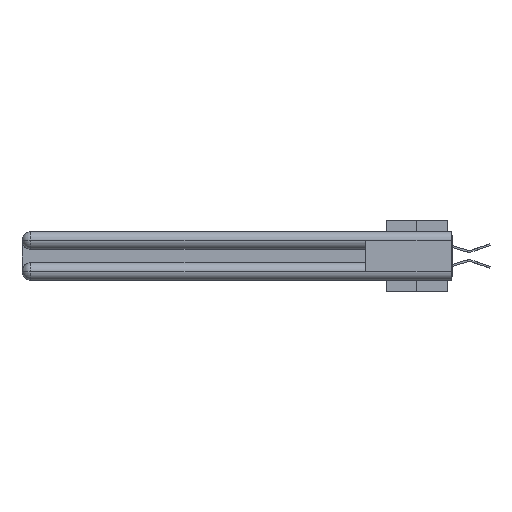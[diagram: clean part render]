
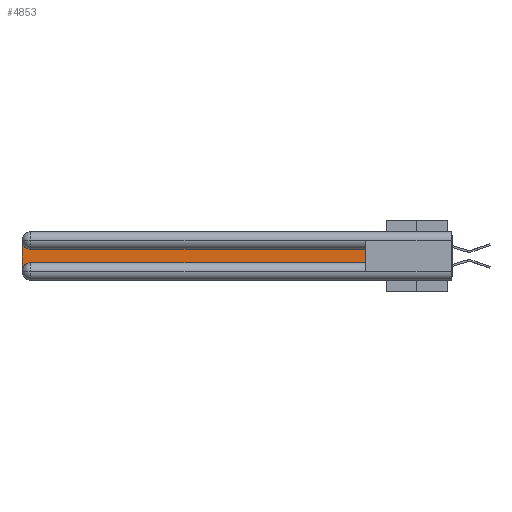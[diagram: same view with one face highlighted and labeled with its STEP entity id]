
A CAD part, left-side view. The second image highlights one B-rep face of the part: STEP entity #4853.
In plain terms, the highlighted planar face has unit normal (-1, 0, 0).
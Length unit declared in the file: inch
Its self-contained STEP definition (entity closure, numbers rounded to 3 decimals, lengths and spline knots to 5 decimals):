
#1683 = CARTESIAN_POINT ( 'NONE',  ( 0.075, 0.6, -0.2175 ) ) ;
#1749 = ORIENTED_EDGE ( 'NONE', *, *, #12714, .T. ) ;
#2126 = DIRECTION ( 'NONE',  ( 0., -1., 0. ) ) ;
#2520 = CARTESIAN_POINT ( 'NONE',  ( 0.075, 0.6, -0.2175 ) ) ;
#4196 = VERTEX_POINT ( 'NONE', #15166 ) ;
#4713 = DIRECTION ( 'NONE',  ( 0., 0., 1. ) ) ;
#4853 = ADVANCED_FACE ( 'NONE', ( #26203 ), #23667, .F. ) ;
#5654 = VERTEX_POINT ( 'NONE', #20560 ) ;
#6648 = LINE ( 'NONE', #21428, #29723 ) ;
#7528 = LINE ( 'NONE', #2520, #30622 ) ;
#7909 = CARTESIAN_POINT ( 'NONE',  ( 0.075, 3., -0.2775 ) ) ;
#9657 = EDGE_CURVE ( 'NONE', #18790, #4196, #7528, .T. ) ;
#10079 = VERTEX_POINT ( 'NONE', #7909 ) ;
#10705 = DIRECTION ( 'NONE',  ( 0., 0., -1. ) ) ;
#11627 = CIRCLE ( 'NONE', #17120, 0.06 ) ;
#12012 = EDGE_CURVE ( 'NONE', #10079, #18790, #11627, .T. ) ;
#12714 = EDGE_CURVE ( 'NONE', #22499, #10079, #35708, .T. ) ;
#13262 = VECTOR ( 'NONE', #4713, 39.37008 ) ;
#13323 = CIRCLE ( 'NONE', #26477, 0.06 ) ;
#13346 = CARTESIAN_POINT ( 'NONE',  ( 0.075, 2.94, -0.0625 ) ) ;
#14436 = VECTOR ( 'NONE', #36068, 39.37008 ) ;
#14522 = EDGE_CURVE ( 'NONE', #4196, #5654, #20319, .T. ) ;
#15166 = CARTESIAN_POINT ( 'NONE',  ( 0.075, 0.6, -0.2175 ) ) ;
#17120 = AXIS2_PLACEMENT_3D ( 'NONE', #26616, #32578, #20451 ) ;
#18790 = VERTEX_POINT ( 'NONE', #24323 ) ;
#19352 = ORIENTED_EDGE ( 'NONE', *, *, #30246, .T. ) ;
#20319 = LINE ( 'NONE', #1683, #13262 ) ;
#20451 = DIRECTION ( 'NONE',  ( 0., 0., -1. ) ) ;
#20560 = CARTESIAN_POINT ( 'NONE',  ( 0.075, 0.6, -0.1225 ) ) ;
#21428 = CARTESIAN_POINT ( 'NONE',  ( 0.075, 0.6, -0.1225 ) ) ;
#22499 = VERTEX_POINT ( 'NONE', #23178 ) ;
#23178 = CARTESIAN_POINT ( 'NONE',  ( 0.075, 3., -0.0625 ) ) ;
#23667 = PLANE ( 'NONE',  #28793 ) ;
#24299 = ORIENTED_EDGE ( 'NONE', *, *, #14522, .T. ) ;
#24323 = CARTESIAN_POINT ( 'NONE',  ( 0.075, 2.94, -0.2175 ) ) ;
#24771 = ORIENTED_EDGE ( 'NONE', *, *, #31123, .T. ) ;
#25160 = DIRECTION ( 'NONE',  ( 1., 0., 0. ) ) ;
#26203 = FACE_OUTER_BOUND ( 'NONE', #29266, .T. ) ;
#26477 = AXIS2_PLACEMENT_3D ( 'NONE', #13346, #25160, #10705 ) ;
#26616 = CARTESIAN_POINT ( 'NONE',  ( 0.075, 2.94, -0.2775 ) ) ;
#28196 = CARTESIAN_POINT ( 'NONE',  ( 0.075, 2.94, -0.1225 ) ) ;
#28793 = AXIS2_PLACEMENT_3D ( 'NONE', #38641, #32550, #39035 ) ;
#29266 = EDGE_LOOP ( 'NONE', ( #24771, #19352, #1749, #32780, #30459, #24299 ) ) ;
#29723 = VECTOR ( 'NONE', #36748, 39.37008 ) ;
#30246 = EDGE_CURVE ( 'NONE', #36396, #22499, #13323, .T. ) ;
#30459 = ORIENTED_EDGE ( 'NONE', *, *, #9657, .T. ) ;
#30622 = VECTOR ( 'NONE', #2126, 39.37008 ) ;
#31123 = EDGE_CURVE ( 'NONE', #5654, #36396, #6648, .T. ) ;
#32550 = DIRECTION ( 'NONE',  ( 1., 0., 0. ) ) ;
#32578 = DIRECTION ( 'NONE',  ( 1., 0., 0. ) ) ;
#32780 = ORIENTED_EDGE ( 'NONE', *, *, #12012, .T. ) ;
#35708 = LINE ( 'NONE', #38886, #14436 ) ;
#36068 = DIRECTION ( 'NONE',  ( 0., 0., -1. ) ) ;
#36396 = VERTEX_POINT ( 'NONE', #28196 ) ;
#36748 = DIRECTION ( 'NONE',  ( 0., 1., 0. ) ) ;
#38641 = CARTESIAN_POINT ( 'NONE',  ( 0.075, 3., -0.1225 ) ) ;
#38886 = CARTESIAN_POINT ( 'NONE',  ( 0.075, 3., -0.2175 ) ) ;
#39035 = DIRECTION ( 'NONE',  ( 0., 0., -1. ) ) ;
